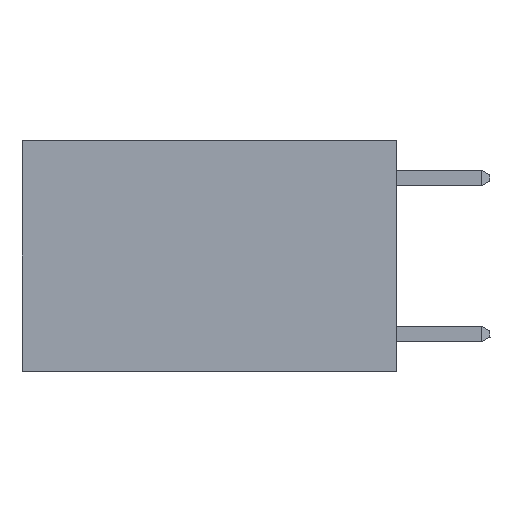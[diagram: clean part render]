
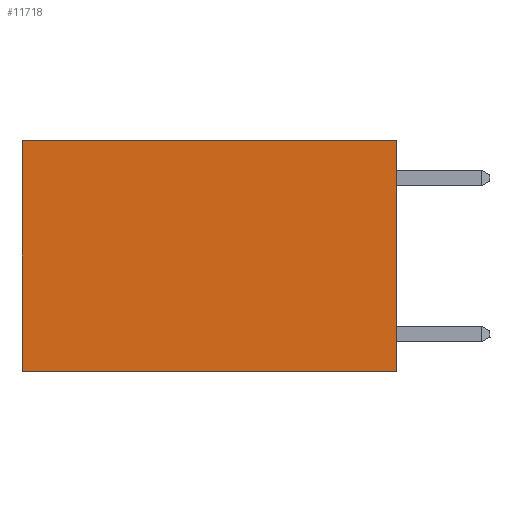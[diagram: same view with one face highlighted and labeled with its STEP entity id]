
A CAD part, left-side view. The second image highlights one B-rep face of the part: STEP entity #11718.
In plain terms, the highlighted planar face has unit normal (-1, 0, 0).
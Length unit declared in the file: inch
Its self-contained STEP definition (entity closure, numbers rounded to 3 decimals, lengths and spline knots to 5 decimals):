
#144 = ORIENTED_EDGE ( 'NONE', *, *, #4190, .T. ) ;
#1608 = CARTESIAN_POINT ( 'NONE',  ( 0.2625, 0., 0. ) ) ;
#1943 = VERTEX_POINT ( 'NONE', #3228 ) ;
#2363 = LINE ( 'NONE', #5277, #12227 ) ;
#2663 = ORIENTED_EDGE ( 'NONE', *, *, #23280, .T. ) ;
#3228 = CARTESIAN_POINT ( 'NONE',  ( 0.2625, 0.6, -0.37 ) ) ;
#3739 = CARTESIAN_POINT ( 'NONE',  ( 0.2625, 0., 0. ) ) ;
#3764 = ORIENTED_EDGE ( 'NONE', *, *, #23800, .F. ) ;
#4190 = EDGE_CURVE ( 'NONE', #20583, #1943, #9611, .T. ) ;
#4902 = LINE ( 'NONE', #3739, #14530 ) ;
#5277 = CARTESIAN_POINT ( 'NONE',  ( 0.2625, 0., -0.37 ) ) ;
#5694 = VERTEX_POINT ( 'NONE', #16349 ) ;
#5783 = DIRECTION ( 'NONE',  ( 0., 0., -1. ) ) ;
#6410 = CARTESIAN_POINT ( 'NONE',  ( 0.2625, 0., 0. ) ) ;
#6927 = VERTEX_POINT ( 'NONE', #11779 ) ;
#7242 = DIRECTION ( 'NONE',  ( 0., 1., 0. ) ) ;
#8369 = DIRECTION ( 'NONE',  ( 1., 0., 0. ) ) ;
#8759 = CARTESIAN_POINT ( 'NONE',  ( 0.2625, 0.6, 0. ) ) ;
#9611 = LINE ( 'NONE', #8759, #9722 ) ;
#9722 = VECTOR ( 'NONE', #21994, 39.37008 ) ;
#9851 = FACE_OUTER_BOUND ( 'NONE', #15293, .T. ) ;
#10024 = CARTESIAN_POINT ( 'NONE',  ( 0.2625, 0.6, 0. ) ) ;
#11718 = ADVANCED_FACE ( 'NONE', ( #9851 ), #19779, .F. ) ;
#11779 = CARTESIAN_POINT ( 'NONE',  ( 0.2625, 0., 0. ) ) ;
#12227 = VECTOR ( 'NONE', #7242, 39.37008 ) ;
#12851 = VECTOR ( 'NONE', #21061, 39.37008 ) ;
#14530 = VECTOR ( 'NONE', #5783, 39.37008 ) ;
#15293 = EDGE_LOOP ( 'NONE', ( #144, #3764, #24818, #2663 ) ) ;
#16349 = CARTESIAN_POINT ( 'NONE',  ( 0.2625, 0., -0.37 ) ) ;
#17551 = EDGE_CURVE ( 'NONE', #6927, #5694, #4902, .T. ) ;
#19618 = AXIS2_PLACEMENT_3D ( 'NONE', #6410, #8369, #21594 ) ;
#19779 = PLANE ( 'NONE',  #19618 ) ;
#20583 = VERTEX_POINT ( 'NONE', #10024 ) ;
#21061 = DIRECTION ( 'NONE',  ( 0., 1., 0. ) ) ;
#21594 = DIRECTION ( 'NONE',  ( 0., 0., -1. ) ) ;
#21994 = DIRECTION ( 'NONE',  ( 0., 0., -1. ) ) ;
#23280 = EDGE_CURVE ( 'NONE', #6927, #20583, #23479, .T. ) ;
#23479 = LINE ( 'NONE', #1608, #12851 ) ;
#23800 = EDGE_CURVE ( 'NONE', #5694, #1943, #2363, .T. ) ;
#24818 = ORIENTED_EDGE ( 'NONE', *, *, #17551, .F. ) ;
